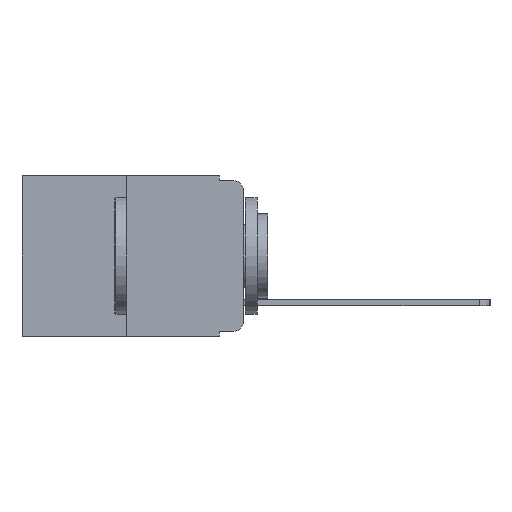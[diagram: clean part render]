
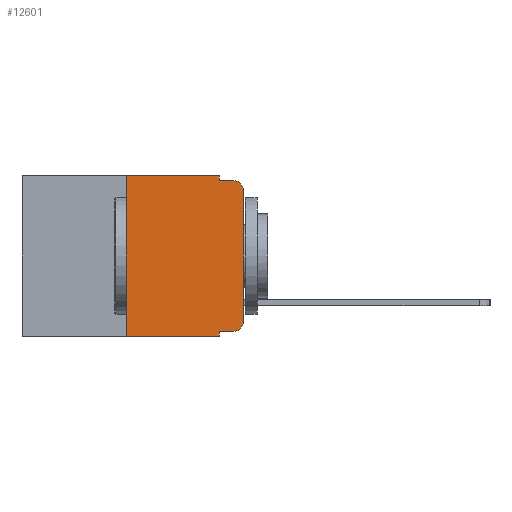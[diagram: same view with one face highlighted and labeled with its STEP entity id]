
A CAD part, left-side view. The second image highlights one B-rep face of the part: STEP entity #12601.
In plain terms, the highlighted planar face has unit normal (-1, 0, 0).
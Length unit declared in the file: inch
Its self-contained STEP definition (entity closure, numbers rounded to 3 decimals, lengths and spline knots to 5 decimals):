
#17 = AXIS2_PLACEMENT_3D ( 'NONE', #23825, #23885, #23861 ) ;
#992 = EDGE_CURVE ( 'NONE', #2185, #1223, #3496, .T. ) ;
#999 = CARTESIAN_POINT ( 'NONE',  ( 0., 0.051, -0.01 ) ) ;
#1223 = VERTEX_POINT ( 'NONE', #23598 ) ;
#1797 = CARTESIAN_POINT ( 'NONE',  ( 0., 0.25, 0. ) ) ;
#1939 = ORIENTED_EDGE ( 'NONE', *, *, #21607, .F. ) ;
#2118 = CIRCLE ( 'NONE', #19540, 0.02 ) ;
#2185 = VERTEX_POINT ( 'NONE', #17863 ) ;
#2220 = LINE ( 'NONE', #23970, #16110 ) ;
#2395 = EDGE_CURVE ( 'NONE', #9853, #2185, #4637, .T. ) ;
#2586 = LINE ( 'NONE', #9366, #7190 ) ;
#2726 = VECTOR ( 'NONE', #14370, 39.37008 ) ;
#3496 = CIRCLE ( 'NONE', #17, 0.02 ) ;
#3502 = VERTEX_POINT ( 'NONE', #13811 ) ;
#4204 = VECTOR ( 'NONE', #8464, 39.37008 ) ;
#4369 = CARTESIAN_POINT ( 'NONE',  ( 0., 0.25, 0. ) ) ;
#4580 = LINE ( 'NONE', #999, #2726 ) ;
#4637 = LINE ( 'NONE', #18912, #18886 ) ;
#4758 = ORIENTED_EDGE ( 'NONE', *, *, #24012, .F. ) ;
#5092 = EDGE_CURVE ( 'NONE', #18250, #21755, #9848, .T. ) ;
#5996 = ORIENTED_EDGE ( 'NONE', *, *, #5092, .F. ) ;
#6191 = FACE_OUTER_BOUND ( 'NONE', #9373, .T. ) ;
#7174 = EDGE_CURVE ( 'NONE', #20294, #7720, #2220, .T. ) ;
#7190 = VECTOR ( 'NONE', #13055, 39.37008 ) ;
#7720 = VERTEX_POINT ( 'NONE', #12552 ) ;
#7955 = CARTESIAN_POINT ( 'NONE',  ( 0., 0.473, 0. ) ) ;
#8349 = ORIENTED_EDGE ( 'NONE', *, *, #19184, .F. ) ;
#8357 = DIRECTION ( 'NONE',  ( -1., 0., 0. ) ) ;
#8401 = VERTEX_POINT ( 'NONE', #19847 ) ;
#8464 = DIRECTION ( 'NONE',  ( 0., -1., 0. ) ) ;
#8639 = ORIENTED_EDGE ( 'NONE', *, *, #2395, .T. ) ;
#8965 = DIRECTION ( 'NONE',  ( 0., 0., 1. ) ) ;
#9366 = CARTESIAN_POINT ( 'NONE',  ( 0., 0.051, -0.333 ) ) ;
#9373 = EDGE_LOOP ( 'NONE', ( #8639, #18996, #4758, #9787, #5996, #1939, #22365, #8349, #18718, #23528 ) ) ;
#9446 = DIRECTION ( 'NONE',  ( 1., 0., 0. ) ) ;
#9503 = AXIS2_PLACEMENT_3D ( 'NONE', #20442, #9446, #22228 ) ;
#9734 = VECTOR ( 'NONE', #15071, 39.37008 ) ;
#9787 = ORIENTED_EDGE ( 'NONE', *, *, #22800, .F. ) ;
#9848 = LINE ( 'NONE', #7955, #4204 ) ;
#9853 = VERTEX_POINT ( 'NONE', #21298 ) ;
#9959 = LINE ( 'NONE', #19635, #14875 ) ;
#10132 = LINE ( 'NONE', #13292, #24124 ) ;
#10301 = CARTESIAN_POINT ( 'NONE',  ( 0., 0.051, 0. ) ) ;
#11174 = CARTESIAN_POINT ( 'NONE',  ( 0., 0.25, -0.343 ) ) ;
#11218 = CARTESIAN_POINT ( 'NONE',  ( 0., 0.051, -0.333 ) ) ;
#12552 = CARTESIAN_POINT ( 'NONE',  ( 0., 0.051, -0.343 ) ) ;
#12601 = ADVANCED_FACE ( 'NONE', ( #6191 ), #23974, .F. ) ;
#13055 = DIRECTION ( 'NONE',  ( 0., -1., 0. ) ) ;
#13292 = CARTESIAN_POINT ( 'NONE',  ( 0., 0.051, 0. ) ) ;
#13811 = CARTESIAN_POINT ( 'NONE',  ( 0., 0.02, -0.333 ) ) ;
#14284 = EDGE_CURVE ( 'NONE', #3502, #9853, #2118, .T. ) ;
#14370 = DIRECTION ( 'NONE',  ( 0., -1., 0. ) ) ;
#14875 = VECTOR ( 'NONE', #21425, 39.37008 ) ;
#15071 = DIRECTION ( 'NONE',  ( 0., 0., 1. ) ) ;
#15168 = DIRECTION ( 'NONE',  ( 0., 0., -1. ) ) ;
#16110 = VECTOR ( 'NONE', #20351, 39.37008 ) ;
#17863 = CARTESIAN_POINT ( 'NONE',  ( 0., 0., -0.03 ) ) ;
#17978 = EDGE_CURVE ( 'NONE', #22414, #3502, #2586, .T. ) ;
#18250 = VERTEX_POINT ( 'NONE', #4369 ) ;
#18718 = ORIENTED_EDGE ( 'NONE', *, *, #17978, .T. ) ;
#18886 = VECTOR ( 'NONE', #8965, 39.37008 ) ;
#18912 = CARTESIAN_POINT ( 'NONE',  ( 0., 0., 0. ) ) ;
#18996 = ORIENTED_EDGE ( 'NONE', *, *, #992, .T. ) ;
#19184 = EDGE_CURVE ( 'NONE', #22414, #7720, #10132, .T. ) ;
#19370 = CARTESIAN_POINT ( 'NONE',  ( 0., 0.02, -0.313 ) ) ;
#19540 = AXIS2_PLACEMENT_3D ( 'NONE', #19370, #8357, #21180 ) ;
#19635 = CARTESIAN_POINT ( 'NONE',  ( 0., 0.051, 0. ) ) ;
#19847 = CARTESIAN_POINT ( 'NONE',  ( 0., 0.051, -0.01 ) ) ;
#20294 = VERTEX_POINT ( 'NONE', #11174 ) ;
#20351 = DIRECTION ( 'NONE',  ( 0., -1., 0. ) ) ;
#20442 = CARTESIAN_POINT ( 'NONE',  ( 0., 0.473, 0. ) ) ;
#21180 = DIRECTION ( 'NONE',  ( 0., 0., -1. ) ) ;
#21298 = CARTESIAN_POINT ( 'NONE',  ( 0., 0., -0.313 ) ) ;
#21425 = DIRECTION ( 'NONE',  ( 0., 0., -1. ) ) ;
#21607 = EDGE_CURVE ( 'NONE', #20294, #18250, #23742, .T. ) ;
#21755 = VERTEX_POINT ( 'NONE', #10301 ) ;
#22228 = DIRECTION ( 'NONE',  ( 0., 0., -1. ) ) ;
#22365 = ORIENTED_EDGE ( 'NONE', *, *, #7174, .T. ) ;
#22414 = VERTEX_POINT ( 'NONE', #11218 ) ;
#22800 = EDGE_CURVE ( 'NONE', #21755, #8401, #9959, .T. ) ;
#23528 = ORIENTED_EDGE ( 'NONE', *, *, #14284, .T. ) ;
#23598 = CARTESIAN_POINT ( 'NONE',  ( 0., 0.02, -0.01 ) ) ;
#23742 = LINE ( 'NONE', #1797, #9734 ) ;
#23825 = CARTESIAN_POINT ( 'NONE',  ( 0., 0.02, -0.03 ) ) ;
#23861 = DIRECTION ( 'NONE',  ( 0., 0., -1. ) ) ;
#23885 = DIRECTION ( 'NONE',  ( -1., 0., 0. ) ) ;
#23970 = CARTESIAN_POINT ( 'NONE',  ( 0., 0.473, -0.343 ) ) ;
#23974 = PLANE ( 'NONE',  #9503 ) ;
#24012 = EDGE_CURVE ( 'NONE', #8401, #1223, #4580, .T. ) ;
#24124 = VECTOR ( 'NONE', #15168, 39.37008 ) ;
